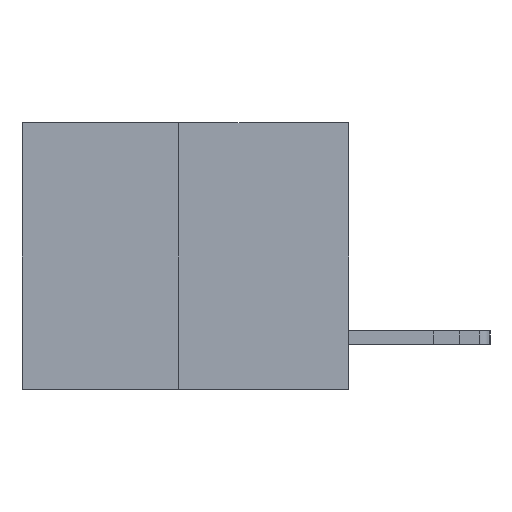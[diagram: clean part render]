
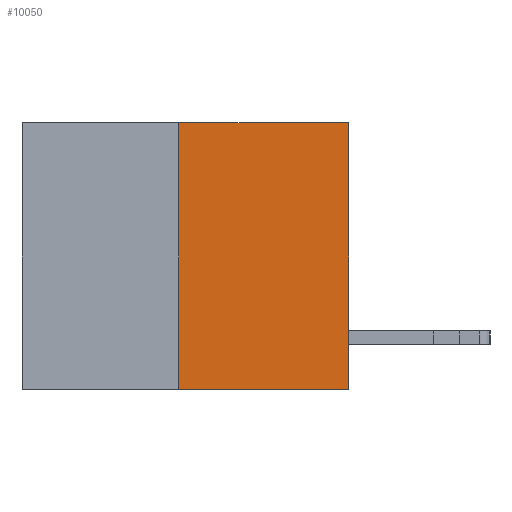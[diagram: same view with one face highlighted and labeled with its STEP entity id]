
A CAD part, left-side view. The second image highlights one B-rep face of the part: STEP entity #10050.
In plain terms, the highlighted planar face has unit normal (-1, 0, 0).
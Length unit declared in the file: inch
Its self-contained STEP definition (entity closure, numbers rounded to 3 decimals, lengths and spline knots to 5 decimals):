
#226 = LINE ( 'NONE', #10738, #3312 ) ;
#636 = CARTESIAN_POINT ( 'NONE',  ( 0., 0.6, -0.49 ) ) ;
#955 = PLANE ( 'NONE',  #18954 ) ;
#1681 = EDGE_CURVE ( 'NONE', #13614, #1961, #15104, .T. ) ;
#1961 = VERTEX_POINT ( 'NONE', #8780 ) ;
#2104 = EDGE_CURVE ( 'NONE', #5851, #1961, #226, .T. ) ;
#2124 = CARTESIAN_POINT ( 'NONE',  ( 0., 0.312, -0.49 ) ) ;
#3169 = VECTOR ( 'NONE', #5061, 39.37008 ) ;
#3312 = VECTOR ( 'NONE', #13692, 39.37008 ) ;
#4111 = CARTESIAN_POINT ( 'NONE',  ( 0., 0.6, 0. ) ) ;
#4654 = CARTESIAN_POINT ( 'NONE',  ( 0., 0., -0.49 ) ) ;
#5061 = DIRECTION ( 'NONE',  ( 0., -1., 0. ) ) ;
#5733 = ORIENTED_EDGE ( 'NONE', *, *, #1681, .F. ) ;
#5813 = ORIENTED_EDGE ( 'NONE', *, *, #10154, .F. ) ;
#5851 = VERTEX_POINT ( 'NONE', #4654 ) ;
#6935 = EDGE_LOOP ( 'NONE', ( #5813, #13061, #17523, #5733 ) ) ;
#6971 = LINE ( 'NONE', #636, #3169 ) ;
#7305 = VECTOR ( 'NONE', #12244, 39.37008 ) ;
#7853 = CARTESIAN_POINT ( 'NONE',  ( 0., 0.312, 0. ) ) ;
#7871 = CARTESIAN_POINT ( 'NONE',  ( 0., 0.312, -0.49 ) ) ;
#8666 = DIRECTION ( 'NONE',  ( 0., 0., -1. ) ) ;
#8780 = CARTESIAN_POINT ( 'NONE',  ( 0., 0., 0. ) ) ;
#10050 = ADVANCED_FACE ( 'NONE', ( #11990 ), #955, .F. ) ;
#10154 = EDGE_CURVE ( 'NONE', #11107, #13614, #10574, .T. ) ;
#10574 = LINE ( 'NONE', #7871, #7305 ) ;
#10738 = CARTESIAN_POINT ( 'NONE',  ( 0., 0., 0. ) ) ;
#11107 = VERTEX_POINT ( 'NONE', #2124 ) ;
#11990 = FACE_OUTER_BOUND ( 'NONE', #6935, .T. ) ;
#12244 = DIRECTION ( 'NONE',  ( 0., 0., 1. ) ) ;
#13061 = ORIENTED_EDGE ( 'NONE', *, *, #13737, .T. ) ;
#13614 = VERTEX_POINT ( 'NONE', #7853 ) ;
#13692 = DIRECTION ( 'NONE',  ( 0., 0., 1. ) ) ;
#13737 = EDGE_CURVE ( 'NONE', #11107, #5851, #6971, .T. ) ;
#14608 = DIRECTION ( 'NONE',  ( 1., 0., 0. ) ) ;
#15104 = LINE ( 'NONE', #19259, #18165 ) ;
#15924 = DIRECTION ( 'NONE',  ( 0., -1., 0. ) ) ;
#17523 = ORIENTED_EDGE ( 'NONE', *, *, #2104, .T. ) ;
#18165 = VECTOR ( 'NONE', #15924, 39.37008 ) ;
#18954 = AXIS2_PLACEMENT_3D ( 'NONE', #4111, #14608, #8666 ) ;
#19259 = CARTESIAN_POINT ( 'NONE',  ( 0., 0.6, 0. ) ) ;
